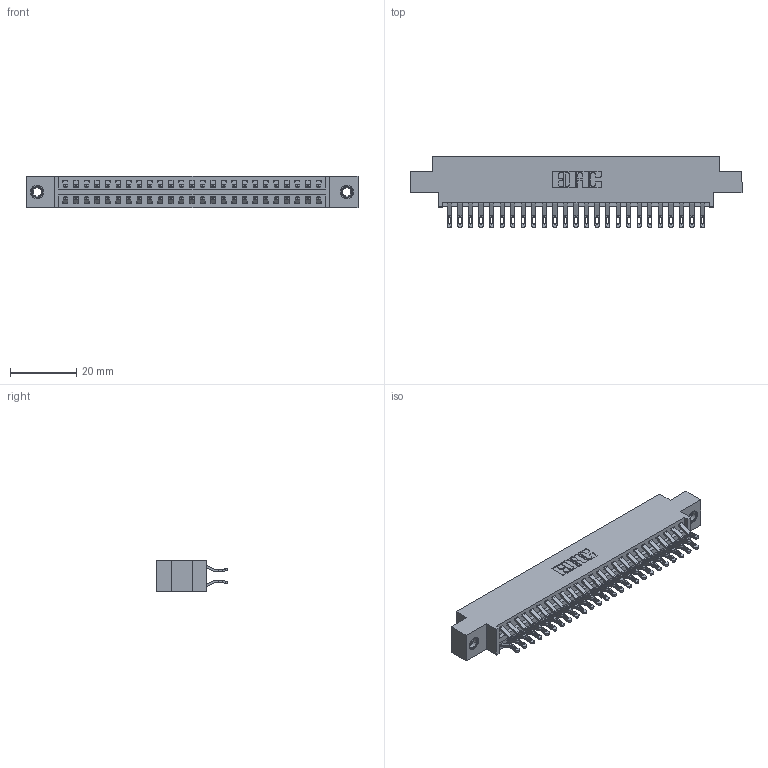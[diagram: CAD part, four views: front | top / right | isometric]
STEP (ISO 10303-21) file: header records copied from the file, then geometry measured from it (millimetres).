
FILE_DESCRIPTION (( 'STEP AP203' ), '1' );
FILE_NAME ('396-050-555-807.STEP', '2019-11-02T07:25:05', ( '' ), ( '' ), 'SwSTEP 2.0', 'SolidWorks 2016', '' );
FILE_SCHEMA (( 'CONFIG_CONTROL_DESIGN' ));
Length unit declared in the file: inch
Products named in the file (4): 346 Part_0.170 Offset - 0.156 Dia-TI; 345-292-001_555 Tail; 345-250-001_345-250-005-103; 396-050-555-807
Assembly tree (53 placements, depth 2):
  396-050-555-807
    346 Part_0.170 Offset - 0.156 Dia-TI
    345-292-001_555 Tail  x50
    345-250-001_345-250-005-103  x2
Bounding box: 99.95 x 21.46 x 9.4 mm (x, y, z)
Volume: 9591.1 mm3; surface area: 13646.8 mm2
Topology: 53 solids, 53 shells, 3086 faces, 9627 edges, 6410 vertices
Faces by surface type: plane 1762, cylinder 1308, cone 12, torus 4
Entity records: 20248 total; most frequent: CARTESIAN_POINT 3381, ORIENTED_EDGE 3278, DIRECTION 3025, EDGE_CURVE 1639, VECTOR 1367, LINE 1367, VERTEX_POINT 1088, AXIS2_PLACEMENT_3D 829
